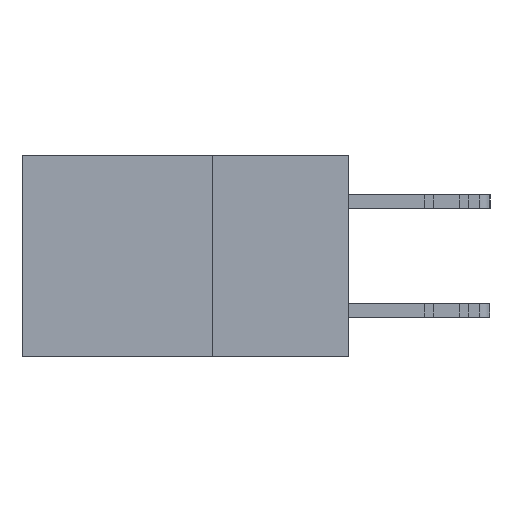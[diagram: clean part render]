
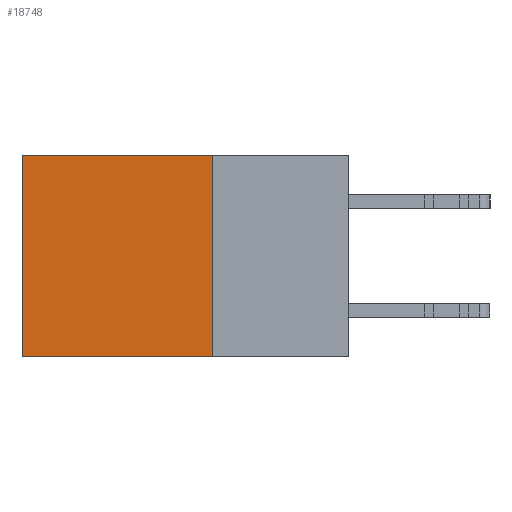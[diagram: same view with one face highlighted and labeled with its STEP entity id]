
A CAD part, left-side view. The second image highlights one B-rep face of the part: STEP entity #18748.
In plain terms, the highlighted planar face has unit normal (-1, 0, 0).
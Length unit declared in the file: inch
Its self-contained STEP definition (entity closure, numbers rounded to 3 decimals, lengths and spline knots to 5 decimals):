
#513 = VECTOR ( 'NONE', #921, 39.37008 ) ;
#921 = DIRECTION ( 'NONE',  ( 0., 0., -1. ) ) ;
#1152 = EDGE_CURVE ( 'NONE', #6968, #24431, #6034, .T. ) ;
#1344 = DIRECTION ( 'NONE',  ( 1., 0., 0. ) ) ;
#1451 = PLANE ( 'NONE',  #28991 ) ;
#3174 = DIRECTION ( 'NONE',  ( 0., 1., 0. ) ) ;
#4196 = DIRECTION ( 'NONE',  ( 0., 0., -1. ) ) ;
#4346 = VECTOR ( 'NONE', #9112, 39.37008 ) ;
#5404 = ORIENTED_EDGE ( 'NONE', *, *, #10514, .T. ) ;
#5927 = CARTESIAN_POINT ( 'NONE',  ( 0.298, 0.25, 0. ) ) ;
#6034 = LINE ( 'NONE', #11576, #4346 ) ;
#6968 = VERTEX_POINT ( 'NONE', #25588 ) ;
#8613 = LINE ( 'NONE', #29166, #28895 ) ;
#9112 = DIRECTION ( 'NONE',  ( 0., 1., 0. ) ) ;
#10514 = EDGE_CURVE ( 'NONE', #20579, #24431, #8613, .T. ) ;
#11576 = CARTESIAN_POINT ( 'NONE',  ( 0.298, 0.25, -0.37 ) ) ;
#12838 = FACE_OUTER_BOUND ( 'NONE', #33141, .T. ) ;
#16598 = ORIENTED_EDGE ( 'NONE', *, *, #1152, .F. ) ;
#16941 = CARTESIAN_POINT ( 'NONE',  ( 0.298, 0.25, 0. ) ) ;
#17101 = DIRECTION ( 'NONE',  ( 0., 0., -1. ) ) ;
#18017 = VECTOR ( 'NONE', #3174, 39.37008 ) ;
#18748 = ADVANCED_FACE ( 'NONE', ( #12838 ), #1451, .F. ) ;
#20093 = ORIENTED_EDGE ( 'NONE', *, *, #31668, .T. ) ;
#20579 = VERTEX_POINT ( 'NONE', #32729 ) ;
#24431 = VERTEX_POINT ( 'NONE', #27293 ) ;
#25588 = CARTESIAN_POINT ( 'NONE',  ( 0.298, 0.25, -0.37 ) ) ;
#25861 = LINE ( 'NONE', #32072, #18017 ) ;
#26829 = ORIENTED_EDGE ( 'NONE', *, *, #27386, .F. ) ;
#27293 = CARTESIAN_POINT ( 'NONE',  ( 0.298, 0.6, -0.37 ) ) ;
#27386 = EDGE_CURVE ( 'NONE', #31042, #6968, #27999, .T. ) ;
#27999 = LINE ( 'NONE', #16941, #513 ) ;
#28895 = VECTOR ( 'NONE', #17101, 39.37008 ) ;
#28991 = AXIS2_PLACEMENT_3D ( 'NONE', #33186, #1344, #4196 ) ;
#29166 = CARTESIAN_POINT ( 'NONE',  ( 0.298, 0.6, 0. ) ) ;
#31042 = VERTEX_POINT ( 'NONE', #5927 ) ;
#31668 = EDGE_CURVE ( 'NONE', #31042, #20579, #25861, .T. ) ;
#32072 = CARTESIAN_POINT ( 'NONE',  ( 0.298, 0.25, 0. ) ) ;
#32729 = CARTESIAN_POINT ( 'NONE',  ( 0.298, 0.6, 0. ) ) ;
#33141 = EDGE_LOOP ( 'NONE', ( #5404, #16598, #26829, #20093 ) ) ;
#33186 = CARTESIAN_POINT ( 'NONE',  ( 0.298, 0.25, 0. ) ) ;
